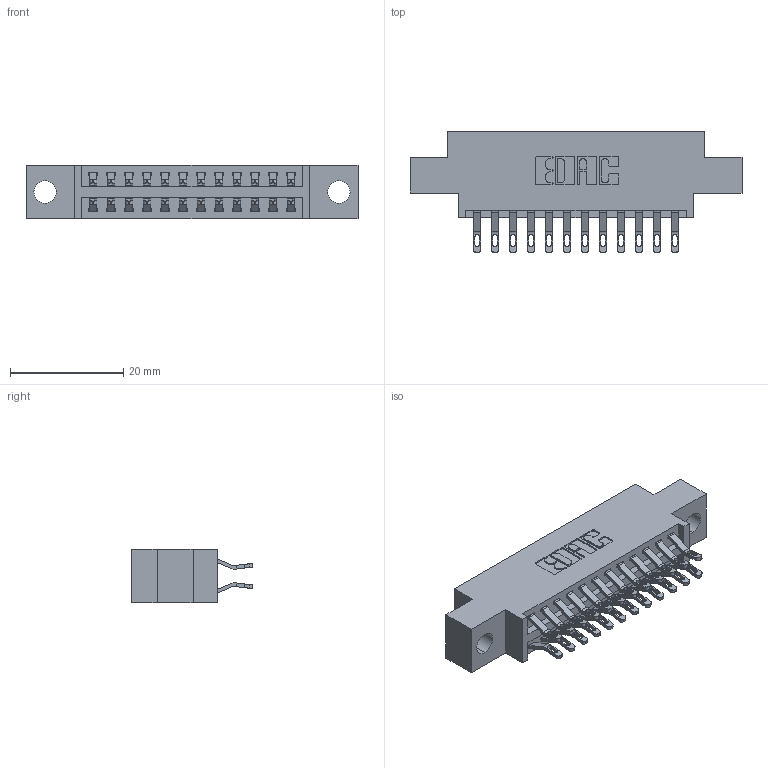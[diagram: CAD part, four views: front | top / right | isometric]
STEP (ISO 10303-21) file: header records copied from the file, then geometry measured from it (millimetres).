
FILE_DESCRIPTION (( 'STEP AP203' ), '1' );
FILE_NAME ('346-024-555-804.STEP', '2022-05-18T23:57:12', ( '' ), ( '' ), 'SwSTEP 2.0', 'SolidWorks 2020', '' );
FILE_SCHEMA (( 'CONFIG_CONTROL_DESIGN' ));
Length unit declared in the file: inch
Products named in the file (3): 345-292-001_555 Tail; 346-024-555-804; 346 Part_0.170 Offset - 0.156 Dia-TH
Assembly tree (25 placements, depth 2):
  346-024-555-804
    346 Part_0.170 Offset - 0.156 Dia-TH
    345-292-001_555 Tail  x24
Bounding box: 58.67 x 21.46 x 9.4 mm (x, y, z)
Volume: 5297.5 mm3; surface area: 7085.9 mm2
Topology: 25 solids, 25 shells, 1532 faces, 4769 edges, 3178 vertices
Faces by surface type: plane 886, cylinder 646
Entity records: 12747 total; most frequent: CARTESIAN_POINT 2184, ORIENTED_EDGE 2086, DIRECTION 1943, EDGE_CURVE 1043, LINE 843, VECTOR 843, VERTEX_POINT 694, AXIS2_PLACEMENT_3D 550
